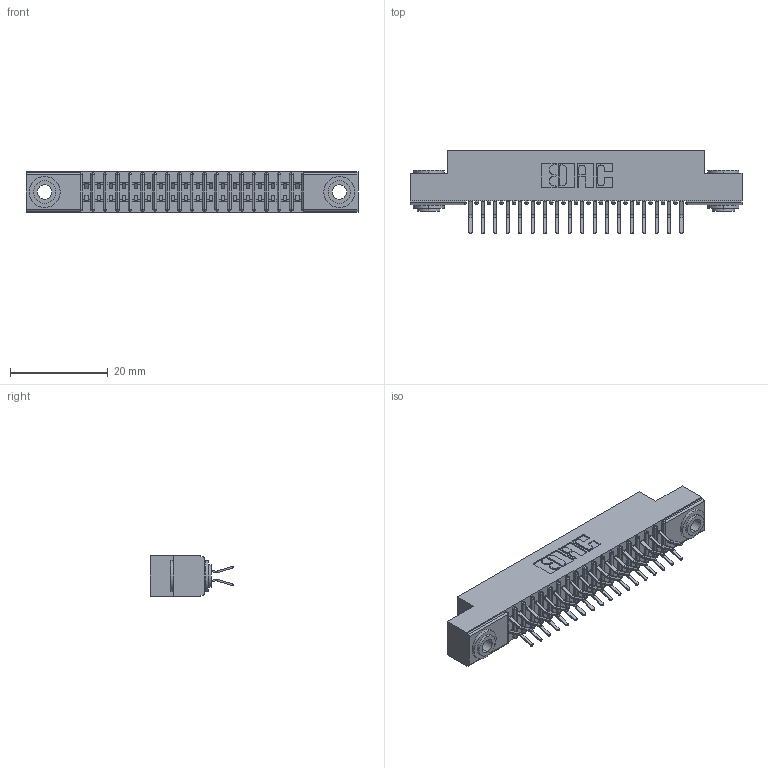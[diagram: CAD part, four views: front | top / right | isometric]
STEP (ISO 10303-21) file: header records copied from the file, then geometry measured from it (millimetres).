
FILE_DESCRIPTION (( 'STEP AP203' ), '1' );
FILE_NAME ('341-036-556-203.STEP', '2018-08-06T22:48:50', ( '' ), ( '' ), 'SwSTEP 2.0', 'SolidWorks 2016', '' );
FILE_SCHEMA (( 'CONFIG_CONTROL_DESIGN' ));
Length unit declared in the file: inch
Products named in the file (4): 345-250-002_345-250-002-102; 341-036-556-203; 341 Part_.156 (3.96) Dia Mounting Holes; 341-292-001_341-292-156
Assembly tree (39 placements, depth 2):
  341-036-556-203
    341 Part_.156 (3.96) Dia Mounting Holes
    341-292-001_341-292-156  x36
    345-250-002_345-250-002-102  x2
Bounding box: 67.94 x 17.07 x 8.38 mm (x, y, z)
Volume: 3891.9 mm3; surface area: 8186 mm2
Topology: 39 solids, 39 shells, 2688 faces, 7754 edges, 5030 vertices
Faces by surface type: plane 1532, cylinder 1076, sphere 38, torus 34, cone 8
Entity records: 26186 total; most frequent: CARTESIAN_POINT 4335, ORIENTED_EDGE 4296, DIRECTION 4244, EDGE_CURVE 2148, LINE 1694, VECTOR 1694, VERTEX_POINT 1366, AXIS2_PLACEMENT_3D 1275
